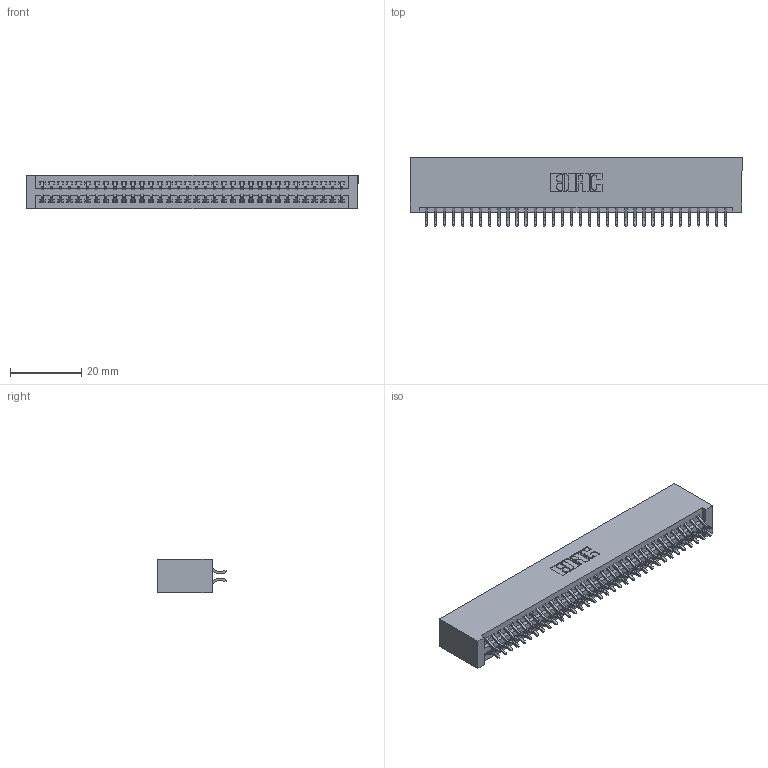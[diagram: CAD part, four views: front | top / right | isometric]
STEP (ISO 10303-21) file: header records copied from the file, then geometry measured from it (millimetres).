
FILE_DESCRIPTION (( 'STEP AP203' ), '1' );
FILE_NAME ('345-068-556-201.STEP', '2019-10-30T21:38:23', ( '' ), ( '' ), 'SwSTEP 2.0', 'SolidWorks 2016', '' );
FILE_SCHEMA (( 'CONFIG_CONTROL_DESIGN' ));
Length unit declared in the file: inch
Products named in the file (3): 345-068-556-201; 345-292-001_556 Tail; 345 Part_No Mounting Lugs
Assembly tree (69 placements, depth 2):
  345-068-556-201
    345 Part_No Mounting Lugs
    345-292-001_556 Tail  x68
Bounding box: 92.96 x 19.24 x 9.4 mm (x, y, z)
Volume: 9569.6 mm3; surface area: 14234.2 mm2
Topology: 69 solids, 69 shells, 3926 faces, 11673 edges, 7690 vertices
Faces by surface type: plane 2592, cylinder 1334
Entity records: 27697 total; most frequent: CARTESIAN_POINT 4664, ORIENTED_EDGE 4586, DIRECTION 4105, EDGE_CURVE 2293, LINE 2025, VECTOR 2025, VERTEX_POINT 1526, AXIS2_PLACEMENT_3D 1040
